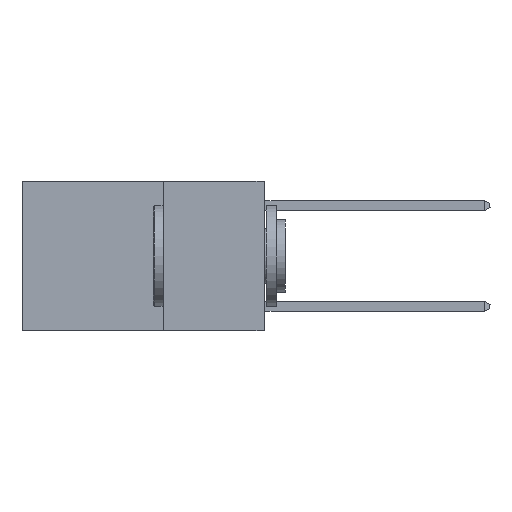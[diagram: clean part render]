
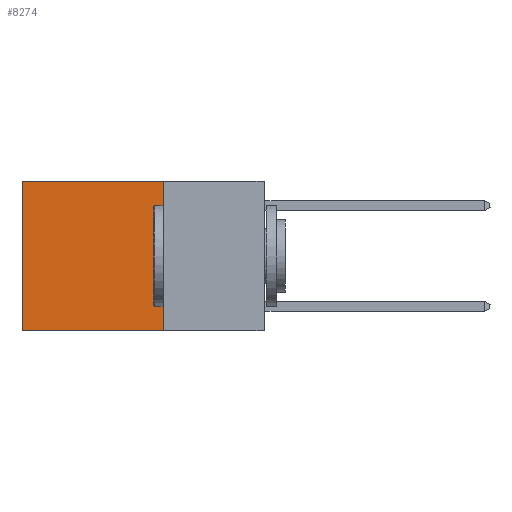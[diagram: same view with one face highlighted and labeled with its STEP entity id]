
A CAD part, left-side view. The second image highlights one B-rep face of the part: STEP entity #8274.
In plain terms, the highlighted planar face has unit normal (-1, 0, 0).
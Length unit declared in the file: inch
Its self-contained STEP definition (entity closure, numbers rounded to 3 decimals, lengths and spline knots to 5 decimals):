
#161 = CARTESIAN_POINT ( 'NONE',  ( 0.2625, 0.25, 0. ) ) ;
#381 = DIRECTION ( 'NONE',  ( 1., 0., 0. ) ) ;
#1028 = EDGE_CURVE ( 'NONE', #10544, #5025, #13150, .T. ) ;
#1433 = PLANE ( 'NONE',  #10069 ) ;
#1996 = DIRECTION ( 'NONE',  ( 0., 0., -1. ) ) ;
#3302 = VECTOR ( 'NONE', #6458, 39.37008 ) ;
#3486 = LINE ( 'NONE', #3573, #5049 ) ;
#3573 = CARTESIAN_POINT ( 'NONE',  ( 0.2625, 0.25, 0. ) ) ;
#3586 = LINE ( 'NONE', #10339, #10872 ) ;
#3606 = LINE ( 'NONE', #15540, #14916 ) ;
#3870 = ORIENTED_EDGE ( 'NONE', *, *, #15706, .F. ) ;
#4037 = CARTESIAN_POINT ( 'NONE',  ( 0.2625, 0.6, 0. ) ) ;
#4635 = ORIENTED_EDGE ( 'NONE', *, *, #16930, .T. ) ;
#4809 = VERTEX_POINT ( 'NONE', #161 ) ;
#5025 = VERTEX_POINT ( 'NONE', #6078 ) ;
#5049 = VECTOR ( 'NONE', #1996, 39.37008 ) ;
#5066 = EDGE_CURVE ( 'NONE', #4809, #7010, #3486, .T. ) ;
#6078 = CARTESIAN_POINT ( 'NONE',  ( 0.2625, 0.6, -0.37 ) ) ;
#6422 = DIRECTION ( 'NONE',  ( 0., 1., 0. ) ) ;
#6458 = DIRECTION ( 'NONE',  ( 0., 0., -1. ) ) ;
#6733 = DIRECTION ( 'NONE',  ( 0., 0., -1. ) ) ;
#6937 = ORIENTED_EDGE ( 'NONE', *, *, #1028, .T. ) ;
#6984 = FACE_OUTER_BOUND ( 'NONE', #15378, .T. ) ;
#7010 = VERTEX_POINT ( 'NONE', #7151 ) ;
#7151 = CARTESIAN_POINT ( 'NONE',  ( 0.2625, 0.25, -0.37 ) ) ;
#8216 = CARTESIAN_POINT ( 'NONE',  ( 0.2625, 0.25, 0. ) ) ;
#8274 = ADVANCED_FACE ( 'NONE', ( #6984 ), #1433, .F. ) ;
#10069 = AXIS2_PLACEMENT_3D ( 'NONE', #8216, #381, #6733 ) ;
#10339 = CARTESIAN_POINT ( 'NONE',  ( 0.2625, 0.25, -0.37 ) ) ;
#10544 = VERTEX_POINT ( 'NONE', #13926 ) ;
#10872 = VECTOR ( 'NONE', #6422, 39.37008 ) ;
#11452 = ORIENTED_EDGE ( 'NONE', *, *, #5066, .F. ) ;
#13150 = LINE ( 'NONE', #4037, #3302 ) ;
#13926 = CARTESIAN_POINT ( 'NONE',  ( 0.2625, 0.6, 0. ) ) ;
#14916 = VECTOR ( 'NONE', #16752, 39.37008 ) ;
#15378 = EDGE_LOOP ( 'NONE', ( #6937, #3870, #11452, #4635 ) ) ;
#15540 = CARTESIAN_POINT ( 'NONE',  ( 0.2625, 0.25, 0. ) ) ;
#15706 = EDGE_CURVE ( 'NONE', #7010, #5025, #3586, .T. ) ;
#16752 = DIRECTION ( 'NONE',  ( 0., 1., 0. ) ) ;
#16930 = EDGE_CURVE ( 'NONE', #4809, #10544, #3606, .T. ) ;
